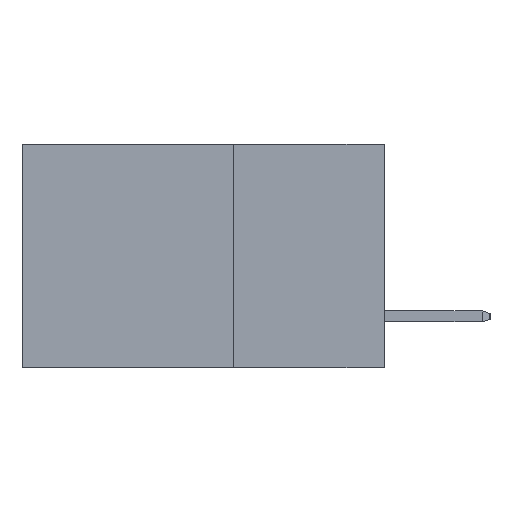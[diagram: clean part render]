
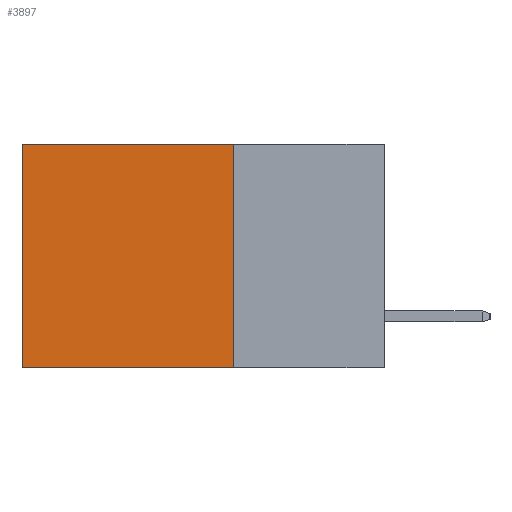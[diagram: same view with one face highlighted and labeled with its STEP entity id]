
A CAD part, left-side view. The second image highlights one B-rep face of the part: STEP entity #3897.
In plain terms, the highlighted planar face has unit normal (-1, 0, 0).
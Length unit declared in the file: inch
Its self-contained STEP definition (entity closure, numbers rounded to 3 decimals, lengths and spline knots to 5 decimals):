
#674 = VERTEX_POINT ( 'NONE', #12790 ) ;
#833 = VECTOR ( 'NONE', #3713, 39.37008 ) ;
#948 = EDGE_LOOP ( 'NONE', ( #1083, #6382, #10348, #3239 ) ) ;
#1083 = ORIENTED_EDGE ( 'NONE', *, *, #7237, .T. ) ;
#1344 = CARTESIAN_POINT ( 'NONE',  ( 0.298, 0.25, 0. ) ) ;
#1381 = VERTEX_POINT ( 'NONE', #6429 ) ;
#2183 = LINE ( 'NONE', #11327, #2929 ) ;
#2929 = VECTOR ( 'NONE', #3429, 39.37008 ) ;
#2932 = PLANE ( 'NONE',  #12923 ) ;
#3011 = EDGE_CURVE ( 'NONE', #1381, #12261, #3492, .T. ) ;
#3239 = ORIENTED_EDGE ( 'NONE', *, *, #3836, .T. ) ;
#3429 = DIRECTION ( 'NONE',  ( 0., 0., -1. ) ) ;
#3492 = LINE ( 'NONE', #4298, #6231 ) ;
#3713 = DIRECTION ( 'NONE',  ( 0., 0., -1. ) ) ;
#3820 = VECTOR ( 'NONE', #6399, 39.37008 ) ;
#3836 = EDGE_CURVE ( 'NONE', #674, #8740, #13090, .T. ) ;
#3897 = ADVANCED_FACE ( 'NONE', ( #9137 ), #2932, .F. ) ;
#4298 = CARTESIAN_POINT ( 'NONE',  ( 0.298, 0.25, -0.37 ) ) ;
#4987 = EDGE_CURVE ( 'NONE', #674, #1381, #6684, .T. ) ;
#6231 = VECTOR ( 'NONE', #14097, 39.37008 ) ;
#6351 = CARTESIAN_POINT ( 'NONE',  ( 0.298, 0.6, 0. ) ) ;
#6382 = ORIENTED_EDGE ( 'NONE', *, *, #3011, .F. ) ;
#6399 = DIRECTION ( 'NONE',  ( 0., 1., 0. ) ) ;
#6429 = CARTESIAN_POINT ( 'NONE',  ( 0.298, 0.25, -0.37 ) ) ;
#6684 = LINE ( 'NONE', #1344, #833 ) ;
#7237 = EDGE_CURVE ( 'NONE', #8740, #12261, #2183, .T. ) ;
#8740 = VERTEX_POINT ( 'NONE', #6351 ) ;
#9137 = FACE_OUTER_BOUND ( 'NONE', #948, .T. ) ;
#10348 = ORIENTED_EDGE ( 'NONE', *, *, #4987, .F. ) ;
#10714 = CARTESIAN_POINT ( 'NONE',  ( 0.298, 0.25, 0. ) ) ;
#11005 = CARTESIAN_POINT ( 'NONE',  ( 0.298, 0.6, -0.37 ) ) ;
#11327 = CARTESIAN_POINT ( 'NONE',  ( 0.298, 0.6, 0. ) ) ;
#12261 = VERTEX_POINT ( 'NONE', #11005 ) ;
#12790 = CARTESIAN_POINT ( 'NONE',  ( 0.298, 0.25, 0. ) ) ;
#12923 = AXIS2_PLACEMENT_3D ( 'NONE', #10714, #13141, #13131 ) ;
#13090 = LINE ( 'NONE', #13892, #3820 ) ;
#13131 = DIRECTION ( 'NONE',  ( 0., 0., -1. ) ) ;
#13141 = DIRECTION ( 'NONE',  ( 1., 0., 0. ) ) ;
#13892 = CARTESIAN_POINT ( 'NONE',  ( 0.298, 0.25, 0. ) ) ;
#14097 = DIRECTION ( 'NONE',  ( 0., 1., 0. ) ) ;
